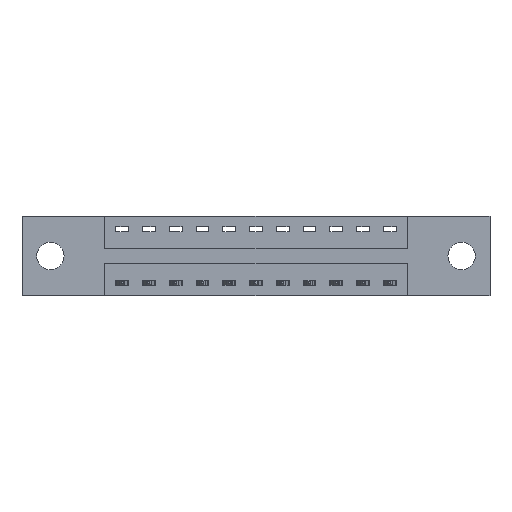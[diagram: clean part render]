
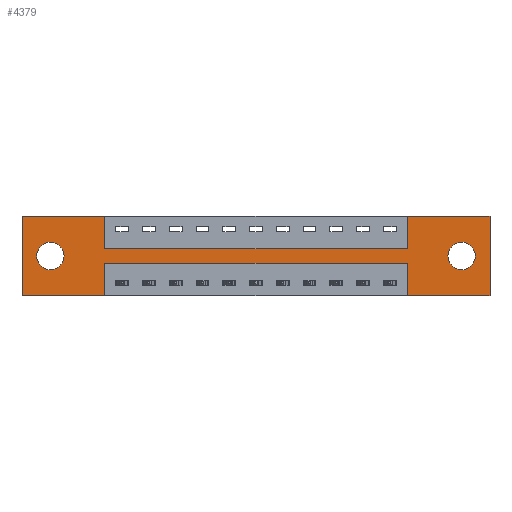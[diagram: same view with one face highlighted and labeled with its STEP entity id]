
A CAD part, front view. The second image highlights one B-rep face of the part: STEP entity #4379.
In plain terms, the highlighted planar face has unit normal (0, -1, 0).
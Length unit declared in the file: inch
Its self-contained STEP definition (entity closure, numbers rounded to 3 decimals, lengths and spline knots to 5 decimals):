
#3 = VERTEX_POINT ( 'NONE', #10847 ) ;
#114 = CARTESIAN_POINT ( 'NONE',  ( 2.185, 0., 0. ) ) ;
#143 = CARTESIAN_POINT ( 'NONE',  ( 0., 0., -0.37 ) ) ;
#362 = DIRECTION ( 'NONE',  ( 0., 0., -1. ) ) ;
#393 = VERTEX_POINT ( 'NONE', #3361 ) ;
#495 = EDGE_CURVE ( 'NONE', #615, #1889, #3602, .T. ) ;
#609 = CARTESIAN_POINT ( 'NONE',  ( 0.1325, 0., -0.185 ) ) ;
#615 = VERTEX_POINT ( 'NONE', #4296 ) ;
#673 = ORIENTED_EDGE ( 'NONE', *, *, #5483, .F. ) ;
#678 = VECTOR ( 'NONE', #10534, 39.37008 ) ;
#863 = VECTOR ( 'NONE', #3980, 39.37008 ) ;
#1078 = CARTESIAN_POINT ( 'NONE',  ( 0.3875, 0., -0.15 ) ) ;
#1138 = LINE ( 'NONE', #4122, #863 ) ;
#1345 = VERTEX_POINT ( 'NONE', #9598 ) ;
#1471 = CARTESIAN_POINT ( 'NONE',  ( 0.1325, 0., -0.185 ) ) ;
#1665 = EDGE_CURVE ( 'NONE', #10393, #8314, #9243, .T. ) ;
#1682 = DIRECTION ( 'NONE',  ( 1., 0., 0. ) ) ;
#1889 = VERTEX_POINT ( 'NONE', #1078 ) ;
#1896 = VECTOR ( 'NONE', #362, 39.37008 ) ;
#1907 = EDGE_CURVE ( 'NONE', #6983, #7564, #5036, .T. ) ;
#2205 = LINE ( 'NONE', #5679, #1896 ) ;
#2490 = VERTEX_POINT ( 'NONE', #5623 ) ;
#2539 = LINE ( 'NONE', #8163, #6896 ) ;
#2553 = ORIENTED_EDGE ( 'NONE', *, *, #495, .F. ) ;
#2559 = CARTESIAN_POINT ( 'NONE',  ( 0., 0., 0. ) ) ;
#2599 = DIRECTION ( 'NONE',  ( 0., 0., 1. ) ) ;
#2606 = DIRECTION ( 'NONE',  ( 0., 1., 0. ) ) ;
#2640 = DIRECTION ( 'NONE',  ( 0., -1., 0. ) ) ;
#2746 = DIRECTION ( 'NONE',  ( 0., 1., 0. ) ) ;
#2846 = FACE_BOUND ( 'NONE', #9559, .T. ) ;
#2863 = CARTESIAN_POINT ( 'NONE',  ( 0., 0., 0. ) ) ;
#3089 = CARTESIAN_POINT ( 'NONE',  ( 0.1325, 0., -0.121 ) ) ;
#3349 = VECTOR ( 'NONE', #7453, 39.37008 ) ;
#3361 = CARTESIAN_POINT ( 'NONE',  ( 1.7975, 0., -0.22 ) ) ;
#3417 = AXIS2_PLACEMENT_3D ( 'NONE', #10138, #2640, #8573 ) ;
#3432 = ORIENTED_EDGE ( 'NONE', *, *, #5743, .T. ) ;
#3483 = EDGE_CURVE ( 'NONE', #7564, #6983, #4297, .T. ) ;
#3542 = EDGE_CURVE ( 'NONE', #10359, #4281, #1138, .T. ) ;
#3591 = VECTOR ( 'NONE', #5258, 39.37008 ) ;
#3602 = LINE ( 'NONE', #7900, #3349 ) ;
#3659 = ORIENTED_EDGE ( 'NONE', *, *, #5419, .F. ) ;
#3838 = VERTEX_POINT ( 'NONE', #4650 ) ;
#3980 = DIRECTION ( 'NONE',  ( 0., 0., 1. ) ) ;
#4093 = AXIS2_PLACEMENT_3D ( 'NONE', #7883, #2746, #8676 ) ;
#4122 = CARTESIAN_POINT ( 'NONE',  ( 1.7975, 0., 0. ) ) ;
#4193 = VECTOR ( 'NONE', #9557, 39.37008 ) ;
#4253 = CARTESIAN_POINT ( 'NONE',  ( 2.0525, 0., -0.185 ) ) ;
#4281 = VERTEX_POINT ( 'NONE', #10040 ) ;
#4296 = CARTESIAN_POINT ( 'NONE',  ( 0.3875, 0., 0. ) ) ;
#4297 = CIRCLE ( 'NONE', #10024, 0.064 ) ;
#4379 = ADVANCED_FACE ( 'NONE', ( #2846, #9568, #5433 ), #7773, .T. ) ;
#4491 = VERTEX_POINT ( 'NONE', #114 ) ;
#4650 = CARTESIAN_POINT ( 'NONE',  ( 2.0525, 0., -0.121 ) ) ;
#4690 = CARTESIAN_POINT ( 'NONE',  ( 2.185, 0., 0. ) ) ;
#4766 = DIRECTION ( 'NONE',  ( -1., 0., 0. ) ) ;
#5001 = CARTESIAN_POINT ( 'NONE',  ( 0., 0., -0.37 ) ) ;
#5036 = CIRCLE ( 'NONE', #9265, 0.064 ) ;
#5116 = ORIENTED_EDGE ( 'NONE', *, *, #9060, .F. ) ;
#5159 = DIRECTION ( 'NONE',  ( 0., 0., -1. ) ) ;
#5169 = DIRECTION ( 'NONE',  ( -1., 0., 0. ) ) ;
#5205 = CARTESIAN_POINT ( 'NONE',  ( 0.3875, 0., -0.15 ) ) ;
#5258 = DIRECTION ( 'NONE',  ( 1., 0., 0. ) ) ;
#5359 = CARTESIAN_POINT ( 'NONE',  ( 0.3875, 0., -0.22 ) ) ;
#5419 = EDGE_CURVE ( 'NONE', #4491, #3, #9797, .T. ) ;
#5433 = FACE_OUTER_BOUND ( 'NONE', #9561, .T. ) ;
#5483 = EDGE_CURVE ( 'NONE', #393, #7199, #2539, .T. ) ;
#5485 = ORIENTED_EDGE ( 'NONE', *, *, #5760, .F. ) ;
#5488 = DIRECTION ( 'NONE',  ( 1., 0., 0. ) ) ;
#5623 = CARTESIAN_POINT ( 'NONE',  ( 2.0525, 0., -0.249 ) ) ;
#5665 = CIRCLE ( 'NONE', #4093, 0.064 ) ;
#5679 = CARTESIAN_POINT ( 'NONE',  ( 0.3875, 0., -0.37 ) ) ;
#5742 = VECTOR ( 'NONE', #1682, 39.37008 ) ;
#5743 = EDGE_CURVE ( 'NONE', #3838, #2490, #11039, .T. ) ;
#5760 = EDGE_CURVE ( 'NONE', #8314, #1345, #8634, .T. ) ;
#5824 = EDGE_CURVE ( 'NONE', #2490, #3838, #5665, .T. ) ;
#5914 = VECTOR ( 'NONE', #5488, 39.37008 ) ;
#5934 = LINE ( 'NONE', #7789, #3591 ) ;
#6024 = LINE ( 'NONE', #9393, #9861 ) ;
#6301 = ORIENTED_EDGE ( 'NONE', *, *, #5824, .T. ) ;
#6522 = ORIENTED_EDGE ( 'NONE', *, *, #10157, .F. ) ;
#6603 = CARTESIAN_POINT ( 'NONE',  ( 0., 0., -0.37 ) ) ;
#6896 = VECTOR ( 'NONE', #4766, 39.37008 ) ;
#6983 = VERTEX_POINT ( 'NONE', #10098 ) ;
#7104 = VECTOR ( 'NONE', #5169, 39.37008 ) ;
#7138 = ORIENTED_EDGE ( 'NONE', *, *, #1665, .F. ) ;
#7199 = VERTEX_POINT ( 'NONE', #5359 ) ;
#7219 = ORIENTED_EDGE ( 'NONE', *, *, #3542, .F. ) ;
#7320 = ORIENTED_EDGE ( 'NONE', *, *, #9503, .F. ) ;
#7453 = DIRECTION ( 'NONE',  ( 0., 0., -1. ) ) ;
#7502 = CARTESIAN_POINT ( 'NONE',  ( 1.7975, 0., -0.37 ) ) ;
#7564 = VERTEX_POINT ( 'NONE', #3089 ) ;
#7597 = DIRECTION ( 'NONE',  ( 0., 1., 0. ) ) ;
#7747 = ORIENTED_EDGE ( 'NONE', *, *, #10112, .F. ) ;
#7750 = ORIENTED_EDGE ( 'NONE', *, *, #1907, .T. ) ;
#7770 = AXIS2_PLACEMENT_3D ( 'NONE', #4253, #10139, #5159 ) ;
#7773 = PLANE ( 'NONE',  #3417 ) ;
#7789 = CARTESIAN_POINT ( 'NONE',  ( 0., 0., 0. ) ) ;
#7883 = CARTESIAN_POINT ( 'NONE',  ( 2.0525, 0., -0.185 ) ) ;
#7888 = DIRECTION ( 'NONE',  ( 0., 0., 1. ) ) ;
#7900 = CARTESIAN_POINT ( 'NONE',  ( 0.3875, 0., 0. ) ) ;
#7926 = EDGE_CURVE ( 'NONE', #1345, #615, #5934, .T. ) ;
#7965 = LINE ( 'NONE', #5205, #5742 ) ;
#8113 = LINE ( 'NONE', #2863, #5914 ) ;
#8163 = CARTESIAN_POINT ( 'NONE',  ( 0.3875, 0., -0.22 ) ) ;
#8314 = VERTEX_POINT ( 'NONE', #6603 ) ;
#8393 = VECTOR ( 'NONE', #2599, 39.37008 ) ;
#8428 = VERTEX_POINT ( 'NONE', #7502 ) ;
#8573 = DIRECTION ( 'NONE',  ( 0., 0., -1. ) ) ;
#8634 = LINE ( 'NONE', #2559, #8393 ) ;
#8676 = DIRECTION ( 'NONE',  ( 0., 0., -1. ) ) ;
#8773 = CARTESIAN_POINT ( 'NONE',  ( 1.7975, 0., -0.15 ) ) ;
#8854 = EDGE_CURVE ( 'NONE', #4281, #4491, #8113, .T. ) ;
#8970 = ORIENTED_EDGE ( 'NONE', *, *, #3483, .T. ) ;
#9060 = EDGE_CURVE ( 'NONE', #7199, #10393, #2205, .T. ) ;
#9243 = LINE ( 'NONE', #5001, #7104 ) ;
#9265 = AXIS2_PLACEMENT_3D ( 'NONE', #1471, #7597, #7888 ) ;
#9361 = DIRECTION ( 'NONE',  ( 0., 0., 1. ) ) ;
#9393 = CARTESIAN_POINT ( 'NONE',  ( 1.7975, 0., -0.37 ) ) ;
#9409 = EDGE_LOOP ( 'NONE', ( #8970, #7750 ) ) ;
#9503 = EDGE_CURVE ( 'NONE', #3, #8428, #10874, .T. ) ;
#9557 = DIRECTION ( 'NONE',  ( -1., 0., 0. ) ) ;
#9559 = EDGE_LOOP ( 'NONE', ( #3432, #6301 ) ) ;
#9561 = EDGE_LOOP ( 'NONE', ( #5116, #673, #6522, #7320, #3659, #9904, #7219, #7747, #2553, #9581, #5485, #7138 ) ) ;
#9568 = FACE_BOUND ( 'NONE', #9409, .T. ) ;
#9581 = ORIENTED_EDGE ( 'NONE', *, *, #7926, .F. ) ;
#9598 = CARTESIAN_POINT ( 'NONE',  ( 0., 0., 0. ) ) ;
#9797 = LINE ( 'NONE', #4690, #678 ) ;
#9861 = VECTOR ( 'NONE', #9361, 39.37008 ) ;
#9904 = ORIENTED_EDGE ( 'NONE', *, *, #8854, .F. ) ;
#10024 = AXIS2_PLACEMENT_3D ( 'NONE', #609, #2606, #10648 ) ;
#10040 = CARTESIAN_POINT ( 'NONE',  ( 1.7975, 0., 0. ) ) ;
#10098 = CARTESIAN_POINT ( 'NONE',  ( 0.1325, 0., -0.249 ) ) ;
#10112 = EDGE_CURVE ( 'NONE', #1889, #10359, #7965, .T. ) ;
#10138 = CARTESIAN_POINT ( 'NONE',  ( 0., 0., -0.37 ) ) ;
#10139 = DIRECTION ( 'NONE',  ( 0., 1., 0. ) ) ;
#10157 = EDGE_CURVE ( 'NONE', #8428, #393, #6024, .T. ) ;
#10359 = VERTEX_POINT ( 'NONE', #8773 ) ;
#10393 = VERTEX_POINT ( 'NONE', #10453 ) ;
#10453 = CARTESIAN_POINT ( 'NONE',  ( 0.3875, 0., -0.37 ) ) ;
#10534 = DIRECTION ( 'NONE',  ( 0., 0., -1. ) ) ;
#10648 = DIRECTION ( 'NONE',  ( 0., 0., 1. ) ) ;
#10847 = CARTESIAN_POINT ( 'NONE',  ( 2.185, 0., -0.37 ) ) ;
#10874 = LINE ( 'NONE', #143, #4193 ) ;
#11039 = CIRCLE ( 'NONE', #7770, 0.064 ) ;
